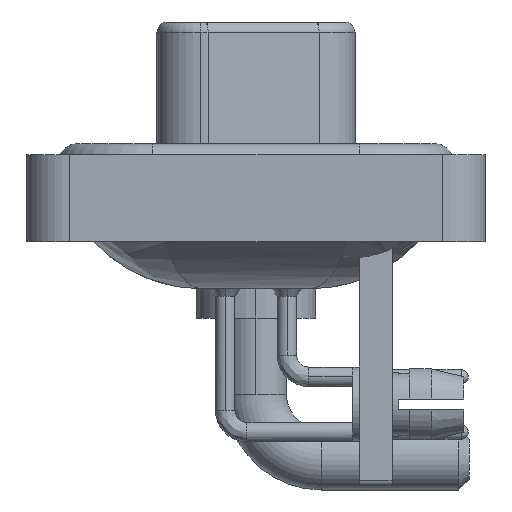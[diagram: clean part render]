
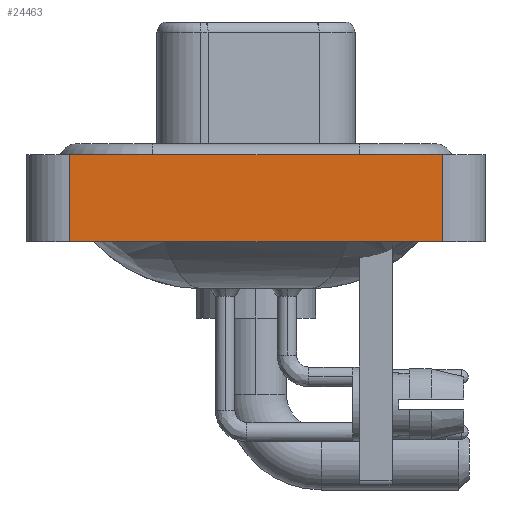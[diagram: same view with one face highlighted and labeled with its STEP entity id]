
A CAD part, left-side view. The second image highlights one B-rep face of the part: STEP entity #24463.
In plain terms, the highlighted planar face has unit normal (-1, 0, 0).
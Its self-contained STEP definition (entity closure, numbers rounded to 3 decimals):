
#319 = CARTESIAN_POINT ( 'NONE',  ( -7.35, -8.55, 0.4 ) ) ;
#1444 = DIRECTION ( 'NONE',  ( -1., 0., 0. ) ) ;
#4326 = CARTESIAN_POINT ( 'NONE',  ( -7.35, 8.55, -3.6 ) ) ;
#4510 = CARTESIAN_POINT ( 'NONE',  ( -7.35, 8.55, -3.6 ) ) ;
#4622 = VECTOR ( 'NONE', #5344, 1000. ) ;
#5344 = DIRECTION ( 'NONE',  ( 0., -1., 0. ) ) ;
#6815 = VECTOR ( 'NONE', #19883, 1000. ) ;
#6998 = ORIENTED_EDGE ( 'NONE', *, *, #9889, .T. ) ;
#7988 = LINE ( 'NONE', #20584, #8694 ) ;
#8694 = VECTOR ( 'NONE', #20753, 1000. ) ;
#9889 = EDGE_CURVE ( 'NONE', #17560, #31331, #15057, .T. ) ;
#12060 = AXIS2_PLACEMENT_3D ( 'NONE', #18263, #1444, #15676 ) ;
#13817 = VERTEX_POINT ( 'NONE', #22988 ) ;
#15057 = LINE ( 'NONE', #24403, #6815 ) ;
#15312 = ORIENTED_EDGE ( 'NONE', *, *, #19659, .T. ) ;
#15538 = LINE ( 'NONE', #319, #4622 ) ;
#15541 = EDGE_CURVE ( 'NONE', #13817, #17744, #15538, .T. ) ;
#15676 = DIRECTION ( 'NONE',  ( 0., 0., 1. ) ) ;
#15716 = VECTOR ( 'NONE', #21933, 1000. ) ;
#16570 = EDGE_LOOP ( 'NONE', ( #15312, #25225, #31538, #6998 ) ) ;
#17560 = VERTEX_POINT ( 'NONE', #4326 ) ;
#17744 = VERTEX_POINT ( 'NONE', #24964 ) ;
#18263 = CARTESIAN_POINT ( 'NONE',  ( -7.35, -8.55, -3.6 ) ) ;
#19659 = EDGE_CURVE ( 'NONE', #31331, #17744, #7988, .T. ) ;
#19883 = DIRECTION ( 'NONE',  ( 0., -1., 0. ) ) ;
#20584 = CARTESIAN_POINT ( 'NONE',  ( -7.35, -8.55, -3.6 ) ) ;
#20753 = DIRECTION ( 'NONE',  ( 0., 0., 1. ) ) ;
#21933 = DIRECTION ( 'NONE',  ( 0., 0., 1. ) ) ;
#22988 = CARTESIAN_POINT ( 'NONE',  ( -7.35, 8.55, 0.4 ) ) ;
#23566 = PLANE ( 'NONE',  #12060 ) ;
#24403 = CARTESIAN_POINT ( 'NONE',  ( -7.35, -8.55, -3.6 ) ) ;
#24463 = ADVANCED_FACE ( 'NONE', ( #28414 ), #23566, .T. ) ;
#24488 = CARTESIAN_POINT ( 'NONE',  ( -7.35, -8.55, -3.6 ) ) ;
#24964 = CARTESIAN_POINT ( 'NONE',  ( -7.35, -8.55, 0.4 ) ) ;
#25025 = EDGE_CURVE ( 'NONE', #17560, #13817, #31298, .T. ) ;
#25225 = ORIENTED_EDGE ( 'NONE', *, *, #15541, .F. ) ;
#28414 = FACE_OUTER_BOUND ( 'NONE', #16570, .T. ) ;
#31298 = LINE ( 'NONE', #4510, #15716 ) ;
#31331 = VERTEX_POINT ( 'NONE', #24488 ) ;
#31538 = ORIENTED_EDGE ( 'NONE', *, *, #25025, .F. ) ;
